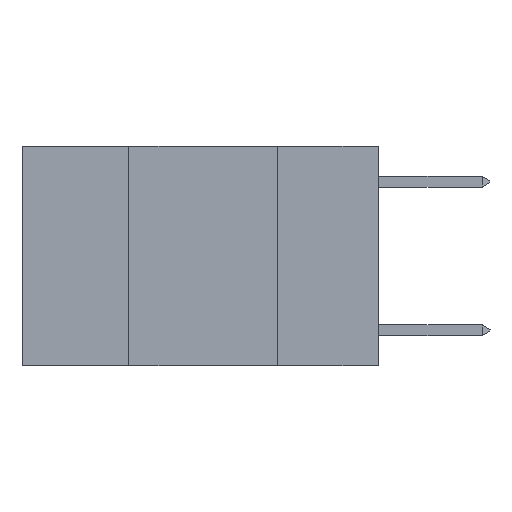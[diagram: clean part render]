
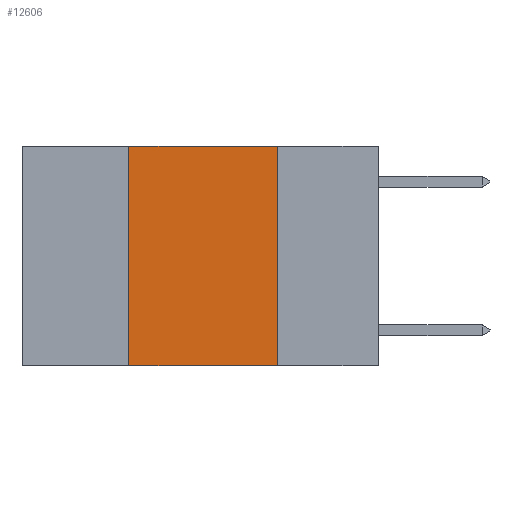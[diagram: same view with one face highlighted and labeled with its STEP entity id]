
A CAD part, left-side view. The second image highlights one B-rep face of the part: STEP entity #12606.
In plain terms, the highlighted planar face has unit normal (-1, 0, 0).
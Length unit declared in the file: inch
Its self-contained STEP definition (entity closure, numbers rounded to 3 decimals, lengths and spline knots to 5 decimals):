
#837 = EDGE_CURVE ( 'NONE', #12115, #10361, #5394, .T. ) ;
#1191 = CARTESIAN_POINT ( 'NONE',  ( 0., 0.42, 0. ) ) ;
#1447 = CARTESIAN_POINT ( 'NONE',  ( 0., 0.42, 0. ) ) ;
#1648 = EDGE_LOOP ( 'NONE', ( #4502, #6225, #12591, #1717 ) ) ;
#1717 = ORIENTED_EDGE ( 'NONE', *, *, #5676, .T. ) ;
#2209 = DIRECTION ( 'NONE',  ( 0., 0., -1. ) ) ;
#2445 = DIRECTION ( 'NONE',  ( 0., 0., 1. ) ) ;
#2546 = DIRECTION ( 'NONE',  ( 0., -1., 0. ) ) ;
#3453 = VECTOR ( 'NONE', #2546, 39.37008 ) ;
#3919 = CARTESIAN_POINT ( 'NONE',  ( 0., 0.17, -0.37 ) ) ;
#4502 = ORIENTED_EDGE ( 'NONE', *, *, #5034, .F. ) ;
#4655 = CARTESIAN_POINT ( 'NONE',  ( 0., 0.42, -0.37 ) ) ;
#5034 = EDGE_CURVE ( 'NONE', #10361, #9573, #12841, .T. ) ;
#5287 = CARTESIAN_POINT ( 'NONE',  ( 0., 0.17, 0. ) ) ;
#5394 = LINE ( 'NONE', #12463, #11316 ) ;
#5676 = EDGE_CURVE ( 'NONE', #8877, #9573, #6626, .T. ) ;
#6225 = ORIENTED_EDGE ( 'NONE', *, *, #837, .F. ) ;
#6626 = LINE ( 'NONE', #7329, #3453 ) ;
#7329 = CARTESIAN_POINT ( 'NONE',  ( 0., 0.6, -0.37 ) ) ;
#8190 = CARTESIAN_POINT ( 'NONE',  ( 0., 0.6, 0. ) ) ;
#8243 = VECTOR ( 'NONE', #2445, 39.37008 ) ;
#8367 = EDGE_CURVE ( 'NONE', #8877, #12115, #11322, .T. ) ;
#8570 = DIRECTION ( 'NONE',  ( 0., 0., -1. ) ) ;
#8586 = AXIS2_PLACEMENT_3D ( 'NONE', #8190, #9335, #2209 ) ;
#8877 = VERTEX_POINT ( 'NONE', #4655 ) ;
#9335 = DIRECTION ( 'NONE',  ( 1., 0., 0. ) ) ;
#9573 = VERTEX_POINT ( 'NONE', #3919 ) ;
#10361 = VERTEX_POINT ( 'NONE', #5287 ) ;
#11316 = VECTOR ( 'NONE', #12027, 39.37008 ) ;
#11322 = LINE ( 'NONE', #1191, #8243 ) ;
#12027 = DIRECTION ( 'NONE',  ( 0., -1., 0. ) ) ;
#12115 = VERTEX_POINT ( 'NONE', #1447 ) ;
#12463 = CARTESIAN_POINT ( 'NONE',  ( 0., 0.6, 0. ) ) ;
#12591 = ORIENTED_EDGE ( 'NONE', *, *, #8367, .F. ) ;
#12606 = ADVANCED_FACE ( 'NONE', ( #15136 ), #13954, .F. ) ;
#12841 = LINE ( 'NONE', #13162, #15187 ) ;
#13162 = CARTESIAN_POINT ( 'NONE',  ( 0., 0.17, 0. ) ) ;
#13954 = PLANE ( 'NONE',  #8586 ) ;
#15136 = FACE_OUTER_BOUND ( 'NONE', #1648, .T. ) ;
#15187 = VECTOR ( 'NONE', #8570, 39.37008 ) ;
